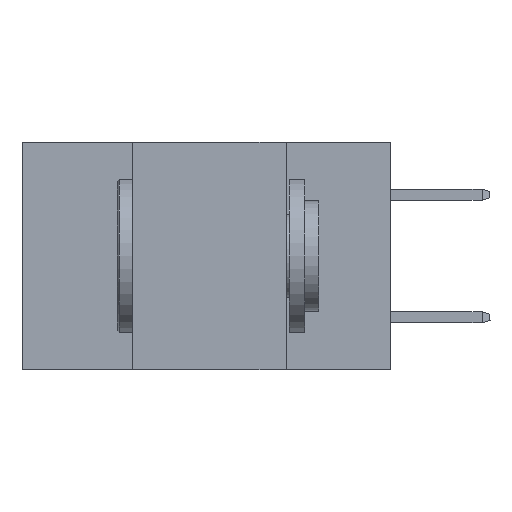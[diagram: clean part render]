
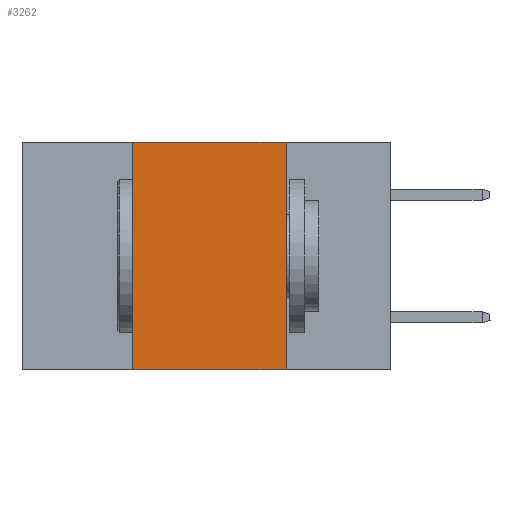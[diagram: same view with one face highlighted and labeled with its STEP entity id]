
A CAD part, left-side view. The second image highlights one B-rep face of the part: STEP entity #3262.
In plain terms, the highlighted planar face has unit normal (-1, 0, 0).
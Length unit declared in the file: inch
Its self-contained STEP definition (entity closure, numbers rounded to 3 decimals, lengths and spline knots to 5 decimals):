
#1297 = VECTOR ( 'NONE', #19985, 39.37008 ) ;
#2128 = CARTESIAN_POINT ( 'NONE',  ( 0., 0.42, 0. ) ) ;
#3262 = ADVANCED_FACE ( 'NONE', ( #36614 ), #10866, .F. ) ;
#3359 = CARTESIAN_POINT ( 'NONE',  ( 0., 0.42, -0.37 ) ) ;
#4362 = CARTESIAN_POINT ( 'NONE',  ( 0., 0.6, 0. ) ) ;
#5402 = AXIS2_PLACEMENT_3D ( 'NONE', #4362, #14138, #36597 ) ;
#5754 = CARTESIAN_POINT ( 'NONE',  ( 0., 0.17, 0. ) ) ;
#6005 = ORIENTED_EDGE ( 'NONE', *, *, #20995, .F. ) ;
#7712 = ORIENTED_EDGE ( 'NONE', *, *, #26787, .F. ) ;
#7739 = CARTESIAN_POINT ( 'NONE',  ( 0., 0.17, -0.37 ) ) ;
#8183 = VERTEX_POINT ( 'NONE', #3359 ) ;
#8713 = CARTESIAN_POINT ( 'NONE',  ( 0., 0.42, 0. ) ) ;
#8767 = EDGE_CURVE ( 'NONE', #8183, #35794, #27074, .T. ) ;
#9896 = LINE ( 'NONE', #16735, #1297 ) ;
#10866 = PLANE ( 'NONE',  #5402 ) ;
#12815 = VERTEX_POINT ( 'NONE', #8713 ) ;
#14078 = EDGE_CURVE ( 'NONE', #23632, #35794, #9896, .T. ) ;
#14138 = DIRECTION ( 'NONE',  ( 1., 0., 0. ) ) ;
#15529 = ORIENTED_EDGE ( 'NONE', *, *, #8767, .T. ) ;
#16735 = CARTESIAN_POINT ( 'NONE',  ( 0., 0.17, 0. ) ) ;
#18505 = VECTOR ( 'NONE', #38192, 39.37008 ) ;
#18867 = EDGE_LOOP ( 'NONE', ( #32492, #7712, #6005, #15529 ) ) ;
#19985 = DIRECTION ( 'NONE',  ( 0., 0., -1. ) ) ;
#20995 = EDGE_CURVE ( 'NONE', #8183, #12815, #37217, .T. ) ;
#23632 = VERTEX_POINT ( 'NONE', #5754 ) ;
#24150 = VECTOR ( 'NONE', #34340, 39.37008 ) ;
#25166 = LINE ( 'NONE', #37379, #24150 ) ;
#25397 = CARTESIAN_POINT ( 'NONE',  ( 0., 0.6, -0.37 ) ) ;
#26787 = EDGE_CURVE ( 'NONE', #12815, #23632, #25166, .T. ) ;
#27074 = LINE ( 'NONE', #25397, #18505 ) ;
#27986 = DIRECTION ( 'NONE',  ( 0., 0., 1. ) ) ;
#28774 = VECTOR ( 'NONE', #27986, 39.37008 ) ;
#32492 = ORIENTED_EDGE ( 'NONE', *, *, #14078, .F. ) ;
#34340 = DIRECTION ( 'NONE',  ( 0., -1., 0. ) ) ;
#35794 = VERTEX_POINT ( 'NONE', #7739 ) ;
#36597 = DIRECTION ( 'NONE',  ( 0., 0., -1. ) ) ;
#36614 = FACE_OUTER_BOUND ( 'NONE', #18867, .T. ) ;
#37217 = LINE ( 'NONE', #2128, #28774 ) ;
#37379 = CARTESIAN_POINT ( 'NONE',  ( 0., 0.6, 0. ) ) ;
#38192 = DIRECTION ( 'NONE',  ( 0., -1., 0. ) ) ;
